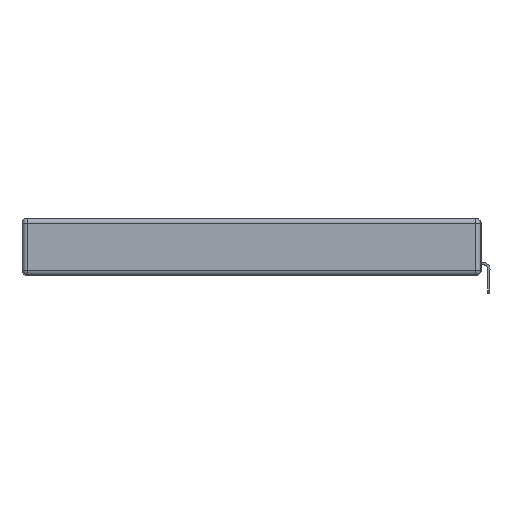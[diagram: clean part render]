
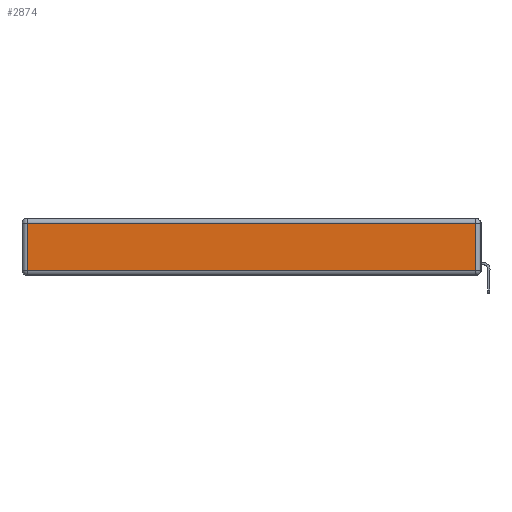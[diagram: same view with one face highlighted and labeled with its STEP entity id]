
A CAD part, left-side view. The second image highlights one B-rep face of the part: STEP entity #2874.
In plain terms, the highlighted planar face has unit normal (-1, 0, 0).
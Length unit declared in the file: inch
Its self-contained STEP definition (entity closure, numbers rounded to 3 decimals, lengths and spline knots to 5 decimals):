
#2534 = VECTOR ( 'NONE', #12019, 39.37008 ) ;
#2745 = DIRECTION ( 'NONE',  ( 0., 0., -1. ) ) ;
#2874 = ADVANCED_FACE ( 'NONE', ( #6817 ), #6630, .T. ) ;
#3150 = LINE ( 'NONE', #12039, #6665 ) ;
#3175 = EDGE_CURVE ( 'NONE', #12635, #7536, #8857, .T. ) ;
#3537 = DIRECTION ( 'NONE',  ( -1., 0., 0. ) ) ;
#3606 = DIRECTION ( 'NONE',  ( 0., -1., 0. ) ) ;
#3699 = CARTESIAN_POINT ( 'NONE',  ( 0., 0.03, -0.343 ) ) ;
#4499 = DIRECTION ( 'NONE',  ( 0., 1., 0. ) ) ;
#4860 = EDGE_LOOP ( 'NONE', ( #11723, #12540, #5333, #12454 ) ) ;
#4913 = EDGE_CURVE ( 'NONE', #9763, #11420, #3150, .T. ) ;
#5333 = ORIENTED_EDGE ( 'NONE', *, *, #3175, .T. ) ;
#5752 = CARTESIAN_POINT ( 'NONE',  ( 0., 2.75, -0.03 ) ) ;
#6353 = LINE ( 'NONE', #10908, #14765 ) ;
#6452 = VECTOR ( 'NONE', #4499, 39.37008 ) ;
#6537 = CARTESIAN_POINT ( 'NONE',  ( 0., 2.72, -0.03 ) ) ;
#6630 = PLANE ( 'NONE',  #9053 ) ;
#6665 = VECTOR ( 'NONE', #3606, 39.37008 ) ;
#6817 = FACE_OUTER_BOUND ( 'NONE', #4860, .T. ) ;
#7536 = VERTEX_POINT ( 'NONE', #6537 ) ;
#8579 = CARTESIAN_POINT ( 'NONE',  ( 0., 0.03, -0.313 ) ) ;
#8857 = LINE ( 'NONE', #5752, #6452 ) ;
#8995 = LINE ( 'NONE', #3699, #2534 ) ;
#9053 = AXIS2_PLACEMENT_3D ( 'NONE', #9236, #3537, #11746 ) ;
#9093 = EDGE_CURVE ( 'NONE', #7536, #9763, #6353, .T. ) ;
#9236 = CARTESIAN_POINT ( 'NONE',  ( 0., 0., -0.343 ) ) ;
#9652 = CARTESIAN_POINT ( 'NONE',  ( 0., 0.03, -0.03 ) ) ;
#9763 = VERTEX_POINT ( 'NONE', #14655 ) ;
#10908 = CARTESIAN_POINT ( 'NONE',  ( 0., 2.72, -0.343 ) ) ;
#11420 = VERTEX_POINT ( 'NONE', #8579 ) ;
#11723 = ORIENTED_EDGE ( 'NONE', *, *, #4913, .T. ) ;
#11746 = DIRECTION ( 'NONE',  ( 0., 0., 1. ) ) ;
#12019 = DIRECTION ( 'NONE',  ( 0., 0., 1. ) ) ;
#12039 = CARTESIAN_POINT ( 'NONE',  ( 0., 0., -0.313 ) ) ;
#12454 = ORIENTED_EDGE ( 'NONE', *, *, #9093, .T. ) ;
#12540 = ORIENTED_EDGE ( 'NONE', *, *, #12649, .T. ) ;
#12635 = VERTEX_POINT ( 'NONE', #9652 ) ;
#12649 = EDGE_CURVE ( 'NONE', #11420, #12635, #8995, .T. ) ;
#14655 = CARTESIAN_POINT ( 'NONE',  ( 0., 2.72, -0.313 ) ) ;
#14765 = VECTOR ( 'NONE', #2745, 39.37008 ) ;
